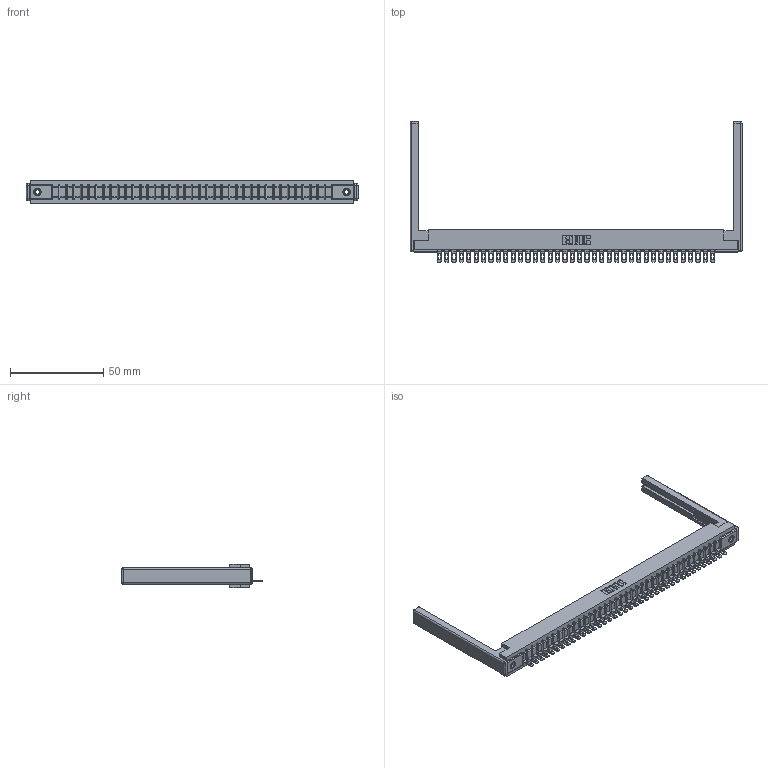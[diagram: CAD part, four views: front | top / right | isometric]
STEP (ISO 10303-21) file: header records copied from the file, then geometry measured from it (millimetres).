
FILE_DESCRIPTION (( 'STEP AP203' ), '1' );
FILE_NAME ('307-038-401-168.STEP', '2020-09-29T06:04:32', ( '' ), ( '' ), 'SwSTEP 2.0', 'SolidWorks 2020', '' );
FILE_SCHEMA (( 'CONFIG_CONTROL_DESIGN' ));
Length unit declared in the file: inch
Products named in the file (5): 345-250-001_345-250-001-102; 307 Part_.156 Dia Mounting Holes; 307-038-401-168; 307-220-068; 307-290-002_501
Assembly tree (43 placements, depth 2):
  307-038-401-168
    307 Part_.156 Dia Mounting Holes
    307-290-002_501  x38
    307-220-068  x2
    345-250-001_345-250-001-102  x2
Bounding box: 178 x 75.39 x 12.7 mm (x, y, z)
Volume: 23429.5 mm3; surface area: 28085.2 mm2
Topology: 43 solids, 43 shells, 3199 faces, 9757 edges, 6378 vertices
Faces by surface type: plane 1830, cylinder 1267, sphere 86, cone 12, torus 4
Entity records: 36623 total; most frequent: CARTESIAN_POINT 6141, ORIENTED_EDGE 6120, DIRECTION 5990, EDGE_CURVE 3060, LINE 2336, VECTOR 2336, VERTEX_POINT 1978, AXIS2_PLACEMENT_3D 1827
